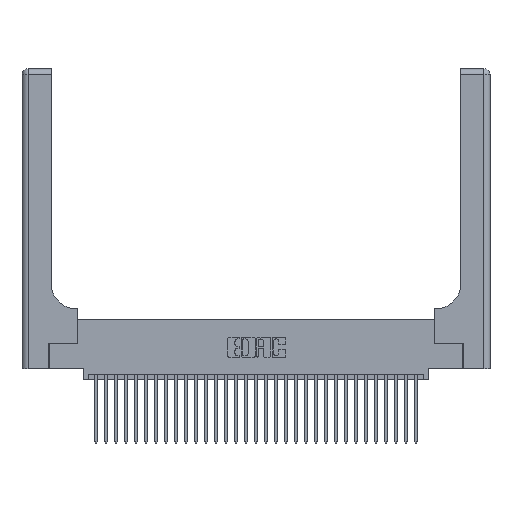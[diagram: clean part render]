
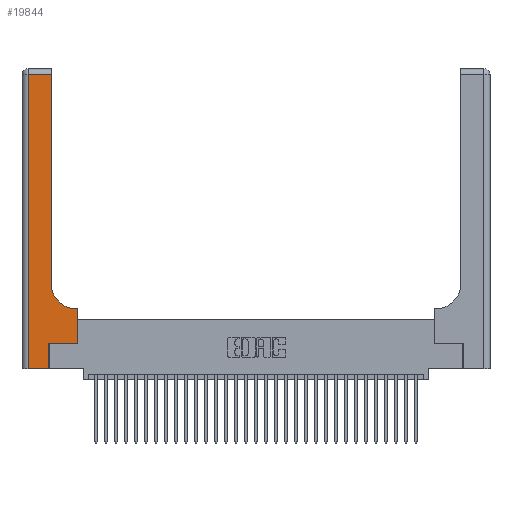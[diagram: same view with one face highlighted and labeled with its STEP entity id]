
A CAD part, top view. The second image highlights one B-rep face of the part: STEP entity #19844.
In plain terms, the highlighted planar face has unit normal (0, 0, 1).
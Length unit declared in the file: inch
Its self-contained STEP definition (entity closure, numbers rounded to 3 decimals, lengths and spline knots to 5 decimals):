
#536 = DIRECTION ( 'NONE',  ( 1., 0., 0. ) ) ;
#629 = VECTOR ( 'NONE', #6344, 39.37008 ) ;
#774 = ORIENTED_EDGE ( 'NONE', *, *, #5771, .T. ) ;
#1398 = CARTESIAN_POINT ( 'NONE',  ( 0.2915, 3., 0.37 ) ) ;
#1934 = VERTEX_POINT ( 'NONE', #14416 ) ;
#2453 = VERTEX_POINT ( 'NONE', #4154 ) ;
#3150 = DIRECTION ( 'NONE',  ( 0., 1., 0. ) ) ;
#3757 = VECTOR ( 'NONE', #26390, 39.37008 ) ;
#4154 = CARTESIAN_POINT ( 'NONE',  ( 0.269, 0.25, 0.37 ) ) ;
#4414 = CARTESIAN_POINT ( 'NONE',  ( 0.2915, 2.94, 0.37 ) ) ;
#5117 = ORIENTED_EDGE ( 'NONE', *, *, #8248, .T. ) ;
#5219 = CARTESIAN_POINT ( 'NONE',  ( 0.269, 0.25, 0.37 ) ) ;
#5493 = VECTOR ( 'NONE', #22236, 39.37008 ) ;
#5722 = CARTESIAN_POINT ( 'NONE',  ( 0.06, 0., 0.37 ) ) ;
#5771 = EDGE_CURVE ( 'NONE', #1934, #11206, #13348, .T. ) ;
#6084 = CARTESIAN_POINT ( 'NONE',  ( 0.5585, 0.6, 0.37 ) ) ;
#6290 = LINE ( 'NONE', #7221, #5493 ) ;
#6344 = DIRECTION ( 'NONE',  ( 0., -1., 0. ) ) ;
#6496 = ORIENTED_EDGE ( 'NONE', *, *, #6643, .T. ) ;
#6643 = EDGE_CURVE ( 'NONE', #23160, #30951, #8949, .T. ) ;
#7107 = EDGE_CURVE ( 'NONE', #14423, #25136, #16362, .T. ) ;
#7221 = CARTESIAN_POINT ( 'NONE',  ( 0., 2.94, 0.37 ) ) ;
#7740 = EDGE_CURVE ( 'NONE', #30951, #30896, #10503, .T. ) ;
#7908 = ORIENTED_EDGE ( 'NONE', *, *, #27957, .T. ) ;
#8248 = EDGE_CURVE ( 'NONE', #2453, #1934, #16336, .T. ) ;
#8695 = LINE ( 'NONE', #12803, #27902 ) ;
#8949 = LINE ( 'NONE', #13936, #629 ) ;
#10503 = LINE ( 'NONE', #18742, #29698 ) ;
#10575 = CARTESIAN_POINT ( 'NONE',  ( 0.269, 0., 0.37 ) ) ;
#11206 = VERTEX_POINT ( 'NONE', #6084 ) ;
#12080 = PLANE ( 'NONE',  #16590 ) ;
#12803 = CARTESIAN_POINT ( 'NONE',  ( 0.269, 0., 0.37 ) ) ;
#13348 = LINE ( 'NONE', #25831, #25094 ) ;
#13479 = EDGE_LOOP ( 'NONE', ( #20900, #31526, #6496, #28994, #7908, #5117, #774, #27665, #24243 ) ) ;
#13696 = VECTOR ( 'NONE', #31389, 39.37008 ) ;
#13936 = CARTESIAN_POINT ( 'NONE',  ( 0.06, 3., 0.37 ) ) ;
#14416 = CARTESIAN_POINT ( 'NONE',  ( 0.5585, 0.25, 0.37 ) ) ;
#14423 = VERTEX_POINT ( 'NONE', #31053 ) ;
#14619 = DIRECTION ( 'NONE',  ( -1., 0., 0. ) ) ;
#15635 = DIRECTION ( 'NONE',  ( 0., 0., -1. ) ) ;
#16252 = DIRECTION ( 'NONE',  ( 1., 0., 0. ) ) ;
#16336 = LINE ( 'NONE', #5219, #23027 ) ;
#16362 = CIRCLE ( 'NONE', #19053, 0.25 ) ;
#16590 = AXIS2_PLACEMENT_3D ( 'NONE', #22040, #29587, #14619 ) ;
#18742 = CARTESIAN_POINT ( 'NONE',  ( 0., 0., 0.37 ) ) ;
#19053 = AXIS2_PLACEMENT_3D ( 'NONE', #30617, #15635, #536 ) ;
#19782 = EDGE_CURVE ( 'NONE', #25136, #20582, #21096, .T. ) ;
#19844 = ADVANCED_FACE ( 'NONE', ( #31235 ), #12080, .F. ) ;
#20210 = DIRECTION ( 'NONE',  ( 1., 0., 0. ) ) ;
#20582 = VERTEX_POINT ( 'NONE', #4414 ) ;
#20900 = ORIENTED_EDGE ( 'NONE', *, *, #19782, .T. ) ;
#21096 = LINE ( 'NONE', #1398, #13696 ) ;
#21099 = EDGE_CURVE ( 'NONE', #11206, #14423, #23046, .T. ) ;
#21988 = CARTESIAN_POINT ( 'NONE',  ( 0.2915, 0.85, 0.37 ) ) ;
#22040 = CARTESIAN_POINT ( 'NONE',  ( 0., 3., 0.37 ) ) ;
#22236 = DIRECTION ( 'NONE',  ( -1., 0., 0. ) ) ;
#23027 = VECTOR ( 'NONE', #20210, 39.37008 ) ;
#23046 = LINE ( 'NONE', #23872, #3757 ) ;
#23160 = VERTEX_POINT ( 'NONE', #26724 ) ;
#23872 = CARTESIAN_POINT ( 'NONE',  ( 0.2915, 0.6, 0.37 ) ) ;
#24243 = ORIENTED_EDGE ( 'NONE', *, *, #7107, .T. ) ;
#25094 = VECTOR ( 'NONE', #3150, 39.37008 ) ;
#25136 = VERTEX_POINT ( 'NONE', #21988 ) ;
#25831 = CARTESIAN_POINT ( 'NONE',  ( 0.5585, 0.25, 0.37 ) ) ;
#26390 = DIRECTION ( 'NONE',  ( -1., 0., 0. ) ) ;
#26724 = CARTESIAN_POINT ( 'NONE',  ( 0.06, 2.94, 0.37 ) ) ;
#27665 = ORIENTED_EDGE ( 'NONE', *, *, #21099, .T. ) ;
#27813 = EDGE_CURVE ( 'NONE', #20582, #23160, #6290, .T. ) ;
#27902 = VECTOR ( 'NONE', #30316, 39.37008 ) ;
#27957 = EDGE_CURVE ( 'NONE', #30896, #2453, #8695, .T. ) ;
#28994 = ORIENTED_EDGE ( 'NONE', *, *, #7740, .T. ) ;
#29587 = DIRECTION ( 'NONE',  ( 0., 0., -1. ) ) ;
#29698 = VECTOR ( 'NONE', #16252, 39.37008 ) ;
#30316 = DIRECTION ( 'NONE',  ( 0., 1., 0. ) ) ;
#30617 = CARTESIAN_POINT ( 'NONE',  ( 0.5415, 0.85, 0.37 ) ) ;
#30896 = VERTEX_POINT ( 'NONE', #10575 ) ;
#30951 = VERTEX_POINT ( 'NONE', #5722 ) ;
#31053 = CARTESIAN_POINT ( 'NONE',  ( 0.5415, 0.6, 0.37 ) ) ;
#31235 = FACE_OUTER_BOUND ( 'NONE', #13479, .T. ) ;
#31389 = DIRECTION ( 'NONE',  ( 0., 1., 0. ) ) ;
#31526 = ORIENTED_EDGE ( 'NONE', *, *, #27813, .T. ) ;
